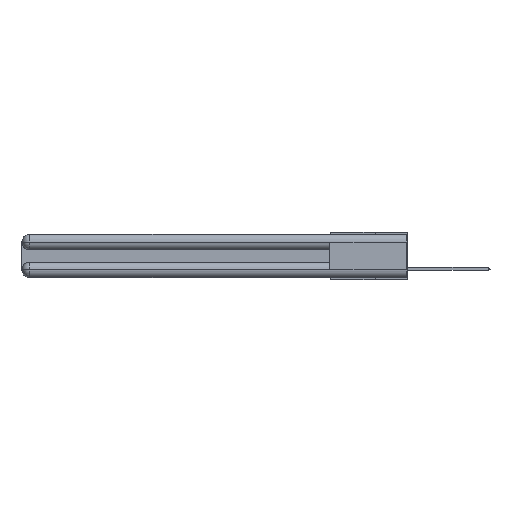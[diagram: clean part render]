
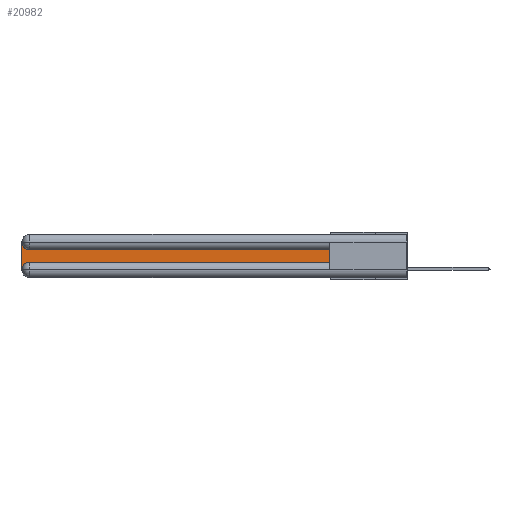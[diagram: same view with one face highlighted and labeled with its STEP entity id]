
A CAD part, left-side view. The second image highlights one B-rep face of the part: STEP entity #20982.
In plain terms, the highlighted planar face has unit normal (-1, 0, 0).
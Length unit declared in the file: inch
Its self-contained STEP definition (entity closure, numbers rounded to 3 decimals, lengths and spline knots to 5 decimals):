
#383 = PLANE ( 'NONE',  #21086 ) ;
#1074 = CARTESIAN_POINT ( 'NONE',  ( 0.075, 3., -0.2175 ) ) ;
#1279 = EDGE_LOOP ( 'NONE', ( #12865, #10584, #19649, #10999, #33468, #15783 ) ) ;
#2695 = CARTESIAN_POINT ( 'NONE',  ( 0.075, 0.6, -0.2175 ) ) ;
#2930 = DIRECTION ( 'NONE',  ( 0., 0., -1. ) ) ;
#4102 = DIRECTION ( 'NONE',  ( 0., 0., -1. ) ) ;
#4643 = CIRCLE ( 'NONE', #14278, 0.06 ) ;
#5460 = CARTESIAN_POINT ( 'NONE',  ( 0.075, 0.6, -0.1225 ) ) ;
#5910 = LINE ( 'NONE', #7583, #8796 ) ;
#6047 = VERTEX_POINT ( 'NONE', #31263 ) ;
#6553 = LINE ( 'NONE', #1074, #28634 ) ;
#7583 = CARTESIAN_POINT ( 'NONE',  ( 0.075, 0.6, -0.2175 ) ) ;
#7691 = CARTESIAN_POINT ( 'NONE',  ( 0.075, 2.94, -0.2775 ) ) ;
#7701 = DIRECTION ( 'NONE',  ( 0., -1., 0. ) ) ;
#8166 = DIRECTION ( 'NONE',  ( 0., 0., -1. ) ) ;
#8301 = VERTEX_POINT ( 'NONE', #5460 ) ;
#8503 = DIRECTION ( 'NONE',  ( 0., 0., -1. ) ) ;
#8581 = DIRECTION ( 'NONE',  ( 0., 1., 0. ) ) ;
#8796 = VECTOR ( 'NONE', #7701, 39.37008 ) ;
#9869 = EDGE_CURVE ( 'NONE', #22215, #8301, #34442, .T. ) ;
#10584 = ORIENTED_EDGE ( 'NONE', *, *, #16969, .T. ) ;
#10745 = DIRECTION ( 'NONE',  ( 1., 0., 0. ) ) ;
#10785 = EDGE_CURVE ( 'NONE', #31058, #22215, #5910, .T. ) ;
#10999 = ORIENTED_EDGE ( 'NONE', *, *, #26164, .T. ) ;
#11466 = CARTESIAN_POINT ( 'NONE',  ( 0.075, 3., -0.0625 ) ) ;
#11553 = VECTOR ( 'NONE', #29488, 39.37008 ) ;
#12465 = LINE ( 'NONE', #27085, #28664 ) ;
#12865 = ORIENTED_EDGE ( 'NONE', *, *, #27772, .T. ) ;
#13688 = CARTESIAN_POINT ( 'NONE',  ( 0.075, 2.94, -0.1225 ) ) ;
#14278 = AXIS2_PLACEMENT_3D ( 'NONE', #7691, #31681, #8166 ) ;
#14971 = CARTESIAN_POINT ( 'NONE',  ( 0.075, 0.6, -0.2175 ) ) ;
#15783 = ORIENTED_EDGE ( 'NONE', *, *, #9869, .T. ) ;
#16969 = EDGE_CURVE ( 'NONE', #23924, #30233, #17314, .T. ) ;
#17314 = CIRCLE ( 'NONE', #26334, 0.06 ) ;
#19649 = ORIENTED_EDGE ( 'NONE', *, *, #33633, .T. ) ;
#20982 = ADVANCED_FACE ( 'NONE', ( #22360 ), #383, .F. ) ;
#21086 = AXIS2_PLACEMENT_3D ( 'NONE', #24141, #10745, #2930 ) ;
#21768 = CARTESIAN_POINT ( 'NONE',  ( 0.075, 2.94, -0.0625 ) ) ;
#22215 = VERTEX_POINT ( 'NONE', #14971 ) ;
#22360 = FACE_OUTER_BOUND ( 'NONE', #1279, .T. ) ;
#23924 = VERTEX_POINT ( 'NONE', #13688 ) ;
#24141 = CARTESIAN_POINT ( 'NONE',  ( 0.075, 3., -0.1225 ) ) ;
#24208 = CARTESIAN_POINT ( 'NONE',  ( 0.075, 2.94, -0.2175 ) ) ;
#24489 = DIRECTION ( 'NONE',  ( 1., 0., 0. ) ) ;
#26164 = EDGE_CURVE ( 'NONE', #6047, #31058, #4643, .T. ) ;
#26334 = AXIS2_PLACEMENT_3D ( 'NONE', #21768, #24489, #8503 ) ;
#27085 = CARTESIAN_POINT ( 'NONE',  ( 0.075, 0.6, -0.1225 ) ) ;
#27772 = EDGE_CURVE ( 'NONE', #8301, #23924, #12465, .T. ) ;
#28634 = VECTOR ( 'NONE', #4102, 39.37008 ) ;
#28664 = VECTOR ( 'NONE', #8581, 39.37008 ) ;
#29488 = DIRECTION ( 'NONE',  ( 0., 0., 1. ) ) ;
#30233 = VERTEX_POINT ( 'NONE', #11466 ) ;
#31058 = VERTEX_POINT ( 'NONE', #24208 ) ;
#31263 = CARTESIAN_POINT ( 'NONE',  ( 0.075, 3., -0.2775 ) ) ;
#31681 = DIRECTION ( 'NONE',  ( 1., 0., 0. ) ) ;
#33468 = ORIENTED_EDGE ( 'NONE', *, *, #10785, .T. ) ;
#33633 = EDGE_CURVE ( 'NONE', #30233, #6047, #6553, .T. ) ;
#34442 = LINE ( 'NONE', #2695, #11553 ) ;
